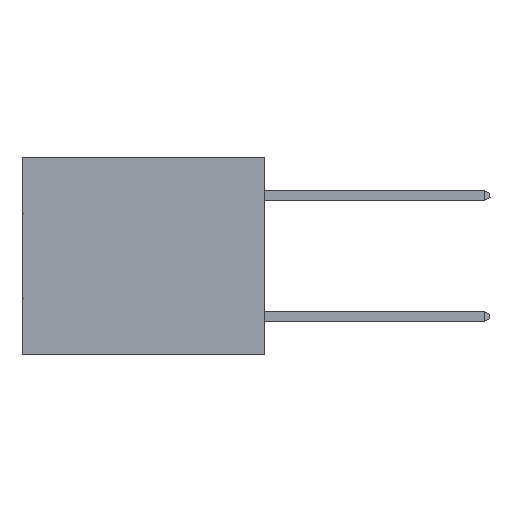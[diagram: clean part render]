
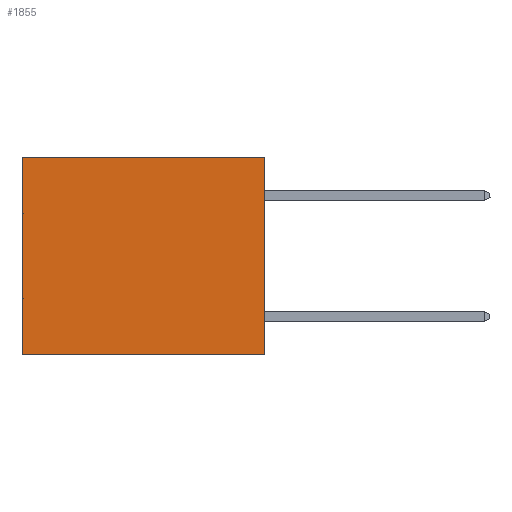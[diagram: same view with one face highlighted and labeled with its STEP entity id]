
A CAD part, left-side view. The second image highlights one B-rep face of the part: STEP entity #1855.
In plain terms, the highlighted planar face has unit normal (-1, 0, 0).
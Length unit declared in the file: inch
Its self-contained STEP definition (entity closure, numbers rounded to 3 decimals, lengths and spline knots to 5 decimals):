
#369 = EDGE_CURVE ( 'NONE', #10210, #22881, #26877, .T. ) ;
#1519 = FACE_OUTER_BOUND ( 'NONE', #4924, .T. ) ;
#1855 = ADVANCED_FACE ( 'NONE', ( #1519 ), #28903, .F. ) ;
#3877 = VERTEX_POINT ( 'NONE', #29195 ) ;
#4924 = EDGE_LOOP ( 'NONE', ( #27814, #5481, #33845, #20912 ) ) ;
#5481 = ORIENTED_EDGE ( 'NONE', *, *, #10680, .F. ) ;
#6634 = VECTOR ( 'NONE', #16986, 39.37008 ) ;
#7705 = VECTOR ( 'NONE', #25234, 39.37008 ) ;
#7786 = CARTESIAN_POINT ( 'NONE',  ( 0.3165, 0., 0. ) ) ;
#9262 = CARTESIAN_POINT ( 'NONE',  ( 0.3165, 0., -0.49 ) ) ;
#9438 = DIRECTION ( 'NONE',  ( 0., 1., 0. ) ) ;
#9702 = VECTOR ( 'NONE', #11429, 39.37008 ) ;
#10210 = VERTEX_POINT ( 'NONE', #7786 ) ;
#10680 = EDGE_CURVE ( 'NONE', #22881, #21564, #16665, .T. ) ;
#11429 = DIRECTION ( 'NONE',  ( 0., 0., -1. ) ) ;
#11528 = CARTESIAN_POINT ( 'NONE',  ( 0.3165, 0., 0. ) ) ;
#12735 = VECTOR ( 'NONE', #9438, 39.37008 ) ;
#15053 = DIRECTION ( 'NONE',  ( 0., 0., -1. ) ) ;
#16369 = AXIS2_PLACEMENT_3D ( 'NONE', #9262, #31473, #15053 ) ;
#16665 = LINE ( 'NONE', #26113, #12735 ) ;
#16986 = DIRECTION ( 'NONE',  ( 0., 1., 0. ) ) ;
#20912 = ORIENTED_EDGE ( 'NONE', *, *, #24227, .T. ) ;
#21564 = VERTEX_POINT ( 'NONE', #32421 ) ;
#22256 = CARTESIAN_POINT ( 'NONE',  ( 0.3165, 0.6, -0.49 ) ) ;
#22319 = CARTESIAN_POINT ( 'NONE',  ( 0.3165, 0., -0.49 ) ) ;
#22881 = VERTEX_POINT ( 'NONE', #33298 ) ;
#24227 = EDGE_CURVE ( 'NONE', #10210, #3877, #25360, .T. ) ;
#25234 = DIRECTION ( 'NONE',  ( 0., 0., -1. ) ) ;
#25360 = LINE ( 'NONE', #11528, #6634 ) ;
#26113 = CARTESIAN_POINT ( 'NONE',  ( 0.3165, 0., -0.49 ) ) ;
#26877 = LINE ( 'NONE', #22319, #7705 ) ;
#27814 = ORIENTED_EDGE ( 'NONE', *, *, #35384, .T. ) ;
#28903 = PLANE ( 'NONE',  #16369 ) ;
#29195 = CARTESIAN_POINT ( 'NONE',  ( 0.3165, 0.6, 0. ) ) ;
#31473 = DIRECTION ( 'NONE',  ( 1., 0., 0. ) ) ;
#31969 = LINE ( 'NONE', #22256, #9702 ) ;
#32421 = CARTESIAN_POINT ( 'NONE',  ( 0.3165, 0.6, -0.49 ) ) ;
#33298 = CARTESIAN_POINT ( 'NONE',  ( 0.3165, 0., -0.49 ) ) ;
#33845 = ORIENTED_EDGE ( 'NONE', *, *, #369, .F. ) ;
#35384 = EDGE_CURVE ( 'NONE', #3877, #21564, #31969, .T. ) ;
